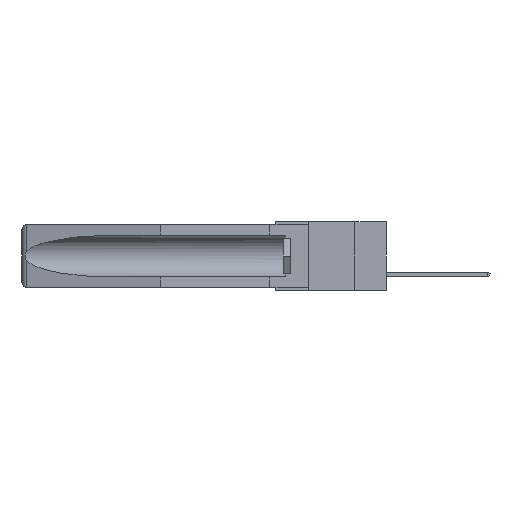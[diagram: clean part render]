
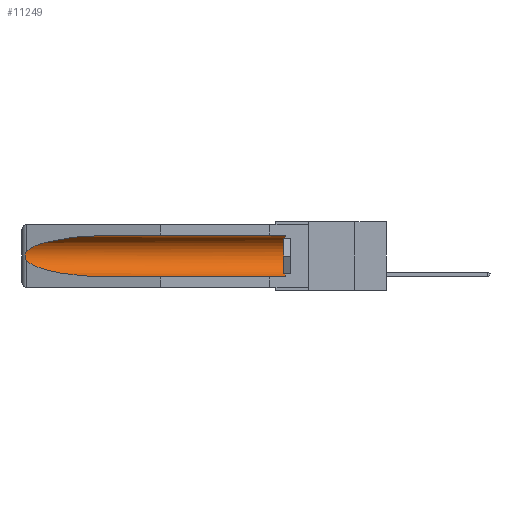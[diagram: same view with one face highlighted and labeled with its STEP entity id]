
A CAD part, left-side view. The second image highlights one B-rep face of the part: STEP entity #11249.
In plain terms, the highlighted cylindrical face has radius 2.857 mm (diameter 5.715 mm), a partial arc.
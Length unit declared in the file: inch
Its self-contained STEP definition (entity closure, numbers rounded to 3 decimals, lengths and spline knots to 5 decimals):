
#26 = CYLINDRICAL_SURFACE ( 'NONE', #30614, 0.1125 ) ;
#890 = ORIENTED_EDGE ( 'NONE', *, *, #11582, .T. ) ;
#1505 = CARTESIAN_POINT ( 'NONE',  ( 0.155, 1.07973, -0.059 ) ) ;
#1815 = CARTESIAN_POINT ( 'NONE',  ( 0.155, 0.126, -0.284 ) ) ;
#2899 = EDGE_LOOP ( 'NONE', ( #890, #25531, #10530, #6438, #18752, #6692 ) ) ;
#3175 = DIRECTION ( 'NONE',  ( 0., 1., 0. ) ) ;
#4896 = CARTESIAN_POINT ( 'NONE',  ( 0.2673, 1.53269, -0.17917 ) ) ;
#6043 = CARTESIAN_POINT ( 'NONE',  ( 0.26537, 1.52718, -0.14972 ) ) ;
#6438 = ORIENTED_EDGE ( 'NONE', *, *, #16495, .F. ) ;
#6692 = ORIENTED_EDGE ( 'NONE', *, *, #28195, .T. ) ;
#7496 = VERTEX_POINT ( 'NONE', #14253 ) ;
#7681 = CARTESIAN_POINT ( 'NONE',  ( 0.155, -0.30754, -0.284 ) ) ;
#8080 = DIRECTION ( 'NONE',  ( 0., 0., 1. ) ) ;
#10518 = CARTESIAN_POINT ( 'NONE',  ( 0.155, -0.30754, -0.059 ) ) ;
#10530 = ORIENTED_EDGE ( 'NONE', *, *, #23139, .T. ) ;
#10616 = DIRECTION ( 'NONE',  ( 0., 0., 1. ) ) ;
#10766 = VERTEX_POINT ( 'NONE', #1815 ) ;
#11249 = ADVANCED_FACE ( 'NONE', ( #21677 ), #26, .F. ) ;
#11582 = EDGE_CURVE ( 'NONE', #13450, #30970, #23031, .T. ) ;
#12032 = CARTESIAN_POINT ( 'NONE',  ( 0.2673, 1.5327, -0.16383 ) ) ;
#12378 = DIRECTION ( 'NONE',  ( 0., 1., 0. ) ) ;
#12675 = AXIS2_PLACEMENT_3D ( 'NONE', #13517, #20991, #10616 ) ;
#13300 = CARTESIAN_POINT ( 'NONE',  ( 0.26537, 1.52718, -0.14972 ) ) ;
#13450 = VERTEX_POINT ( 'NONE', #1505 ) ;
#13517 = CARTESIAN_POINT ( 'NONE',  ( 0.155, 0.126, -0.1715 ) ) ;
#14253 = CARTESIAN_POINT ( 'NONE',  ( 0.26537, 1.52718, -0.19328 ) ) ;
#16211 = CIRCLE ( 'NONE', #12675, 0.1125 ) ;
#16297 = VERTEX_POINT ( 'NONE', #17451 ) ;
#16495 = EDGE_CURVE ( 'NONE', #10766, #16297, #31378, .T. ) ;
#16696 = LINE ( 'NONE', #10518, #21140 ) ;
#17451 = CARTESIAN_POINT ( 'NONE',  ( 0.155, 1.07973, -0.284 ) ) ;
#18616 = B_SPLINE_CURVE_WITH_KNOTS ( 'NONE', 3,
 ( #32466, #19709, #27390, #12032, #32572, #20269, #4896, #20386, #27961, #20161 ),
 .UNSPECIFIED., .F., .F.,
 ( 4, 2, 2, 2, 4 ),
 ( 0., 0.00029, 0.00058, 0.00087, 0.00117 ),
 .UNSPECIFIED. ) ;
#18752 = ORIENTED_EDGE ( 'NONE', *, *, #29941, .T. ) ;
#19709 = CARTESIAN_POINT ( 'NONE',  ( 0.26597, 1.52961, -0.15275 ) ) ;
#20085 =( BOUNDED_CURVE ( )  B_SPLINE_CURVE ( 3, ( #26919, #26582, #29162, #29494 ),
 .UNSPECIFIED., .F., .F. ) 
 B_SPLINE_CURVE_WITH_KNOTS ( ( 4, 4 ),
 ( 0.1948, 1.5708 ),
 .UNSPECIFIED. ) 
 CURVE ( )  GEOMETRIC_REPRESENTATION_ITEM ( )  RATIONAL_B_SPLINE_CURVE ( ( 1., 0.848, 0.848, 1. ) ) 
 REPRESENTATION_ITEM ( '' )  );
#20161 = CARTESIAN_POINT ( 'NONE',  ( 0.26537, 1.52718, -0.19328 ) ) ;
#20269 = CARTESIAN_POINT ( 'NONE',  ( 0.2675, 1.53308, -0.17534 ) ) ;
#20386 = CARTESIAN_POINT ( 'NONE',  ( 0.26655, 1.53094, -0.18657 ) ) ;
#20434 = CARTESIAN_POINT ( 'NONE',  ( 0.155, 0.126, -0.059 ) ) ;
#20895 = VERTEX_POINT ( 'NONE', #20434 ) ;
#20991 = DIRECTION ( 'NONE',  ( 0., -1., 0. ) ) ;
#21140 = VECTOR ( 'NONE', #26527, 39.37008 ) ;
#21383 = EDGE_CURVE ( 'NONE', #30970, #7496, #18616, .T. ) ;
#21413 = CARTESIAN_POINT ( 'NONE',  ( 0.155, 1.07973, -0.059 ) ) ;
#21677 = FACE_OUTER_BOUND ( 'NONE', #2899, .T. ) ;
#23031 =( BOUNDED_CURVE ( )  B_SPLINE_CURVE ( 3, ( #21413, #32029, #29218, #6043 ),
 .UNSPECIFIED., .F., .F. ) 
 B_SPLINE_CURVE_WITH_KNOTS ( ( 4, 4 ),
 ( 4.71239, 6.08839 ),
 .UNSPECIFIED. ) 
 CURVE ( )  GEOMETRIC_REPRESENTATION_ITEM ( )  RATIONAL_B_SPLINE_CURVE ( ( 1., 0.848, 0.848, 1. ) ) 
 REPRESENTATION_ITEM ( '' )  );
#23139 = EDGE_CURVE ( 'NONE', #7496, #16297, #20085, .T. ) ;
#23476 = CARTESIAN_POINT ( 'NONE',  ( 0.155, -0.30754, -0.1715 ) ) ;
#23779 = VECTOR ( 'NONE', #12378, 39.37008 ) ;
#25531 = ORIENTED_EDGE ( 'NONE', *, *, #21383, .T. ) ;
#26527 = DIRECTION ( 'NONE',  ( 0., 1., 0. ) ) ;
#26582 = CARTESIAN_POINT ( 'NONE',  ( 0.25451, 1.48313, -0.24835 ) ) ;
#26919 = CARTESIAN_POINT ( 'NONE',  ( 0.26537, 1.52718, -0.19328 ) ) ;
#27390 = CARTESIAN_POINT ( 'NONE',  ( 0.26654, 1.53092, -0.15636 ) ) ;
#27961 = CARTESIAN_POINT ( 'NONE',  ( 0.26597, 1.5296, -0.19026 ) ) ;
#28195 = EDGE_CURVE ( 'NONE', #20895, #13450, #16696, .T. ) ;
#29162 = CARTESIAN_POINT ( 'NONE',  ( 0.21114, 1.30732, -0.284 ) ) ;
#29218 = CARTESIAN_POINT ( 'NONE',  ( 0.25451, 1.48313, -0.09465 ) ) ;
#29494 = CARTESIAN_POINT ( 'NONE',  ( 0.155, 1.07973, -0.284 ) ) ;
#29941 = EDGE_CURVE ( 'NONE', #10766, #20895, #16211, .T. ) ;
#30614 = AXIS2_PLACEMENT_3D ( 'NONE', #23476, #3175, #8080 ) ;
#30970 = VERTEX_POINT ( 'NONE', #13300 ) ;
#31378 = LINE ( 'NONE', #7681, #23779 ) ;
#32029 = CARTESIAN_POINT ( 'NONE',  ( 0.21114, 1.30732, -0.059 ) ) ;
#32466 = CARTESIAN_POINT ( 'NONE',  ( 0.26537, 1.52718, -0.14972 ) ) ;
#32572 = CARTESIAN_POINT ( 'NONE',  ( 0.2675, 1.53308, -0.16763 ) ) ;
